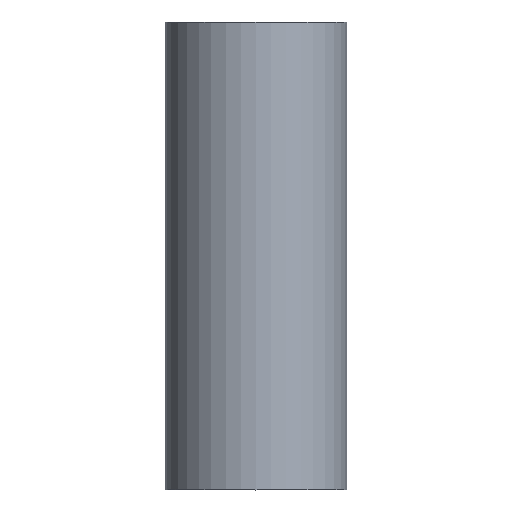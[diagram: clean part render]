
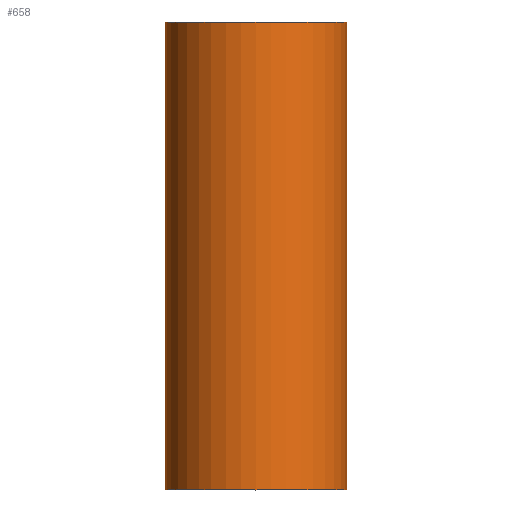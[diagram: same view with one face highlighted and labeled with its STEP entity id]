
A CAD part, front view. The second image highlights one B-rep face of the part: STEP entity #658.
In plain terms, the highlighted cylindrical face has radius 18.575 mm (diameter 37.15 mm), a partial arc.
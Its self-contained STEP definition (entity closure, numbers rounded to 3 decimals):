
#35 = CARTESIAN_POINT ( 'NONE',  ( 12.715, 43.749, -9.184 ) ) ;
#102 = EDGE_CURVE ( 'NONE', #840, #176, #2010, .T. ) ;
#111 = CARTESIAN_POINT ( 'NONE',  ( 12.715, 43.749, 31.866 ) ) ;
#155 = AXIS2_PLACEMENT_3D ( 'NONE', #1401, #329, #1579 ) ;
#163 = ORIENTED_EDGE ( 'NONE', *, *, #1906, .T. ) ;
#165 = EDGE_LOOP ( 'NONE', ( #1978, #1896, #163, #900 ) ) ;
#176 = VERTEX_POINT ( 'NONE', #964 ) ;
#203 = DIRECTION ( 'NONE',  ( 0., 0., 1. ) ) ;
#246 = FACE_OUTER_BOUND ( 'NONE', #165, .T. ) ;
#277 = VECTOR ( 'NONE', #1821, 1000. ) ;
#287 = AXIS2_PLACEMENT_3D ( 'NONE', #111, #1356, #311 ) ;
#311 = DIRECTION ( 'NONE',  ( 1., 0., 0. ) ) ;
#329 = DIRECTION ( 'NONE',  ( 0., 0., -1. ) ) ;
#464 = CARTESIAN_POINT ( 'NONE',  ( 31.282, 43.19, 127.673 ) ) ;
#502 = VERTEX_POINT ( 'NONE', #1803 ) ;
#643 = CIRCLE ( 'NONE', #155, 18.575 ) ;
#658 = ADVANCED_FACE ( 'NONE', ( #246 ), #1726, .T. ) ;
#734 = CIRCLE ( 'NONE', #287, 18.575 ) ;
#840 = VERTEX_POINT ( 'NONE', #1645 ) ;
#900 = ORIENTED_EDGE ( 'NONE', *, *, #2145, .T. ) ;
#964 = CARTESIAN_POINT ( 'NONE',  ( -5.851, 43.19, 127.673 ) ) ;
#981 = VERTEX_POINT ( 'NONE', #464 ) ;
#1023 = AXIS2_PLACEMENT_3D ( 'NONE', #35, #1835, #1884 ) ;
#1219 = LINE ( 'NONE', #1642, #277 ) ;
#1356 = DIRECTION ( 'NONE',  ( 0., 0., -1. ) ) ;
#1394 = CARTESIAN_POINT ( 'NONE',  ( -5.851, 43.19, 278.475 ) ) ;
#1401 = CARTESIAN_POINT ( 'NONE',  ( 12.715, 43.749, 127.673 ) ) ;
#1545 = VECTOR ( 'NONE', #203, 1000. ) ;
#1579 = DIRECTION ( 'NONE',  ( -1., 0., 0. ) ) ;
#1642 = CARTESIAN_POINT ( 'NONE',  ( 31.282, 43.19, 278.475 ) ) ;
#1645 = CARTESIAN_POINT ( 'NONE',  ( -5.851, 43.19, 31.866 ) ) ;
#1726 = CYLINDRICAL_SURFACE ( 'NONE', #1023, 18.575 ) ;
#1803 = CARTESIAN_POINT ( 'NONE',  ( 31.282, 43.19, 31.866 ) ) ;
#1821 = DIRECTION ( 'NONE',  ( 0., 0., 1. ) ) ;
#1835 = DIRECTION ( 'NONE',  ( 0., 0., 1. ) ) ;
#1884 = DIRECTION ( 'NONE',  ( -1., 0., 0. ) ) ;
#1896 = ORIENTED_EDGE ( 'NONE', *, *, #1994, .F. ) ;
#1906 = EDGE_CURVE ( 'NONE', #502, #981, #1219, .T. ) ;
#1978 = ORIENTED_EDGE ( 'NONE', *, *, #102, .F. ) ;
#1994 = EDGE_CURVE ( 'NONE', #502, #840, #734, .T. ) ;
#2010 = LINE ( 'NONE', #1394, #1545 ) ;
#2145 = EDGE_CURVE ( 'NONE', #981, #176, #643, .T. ) ;
